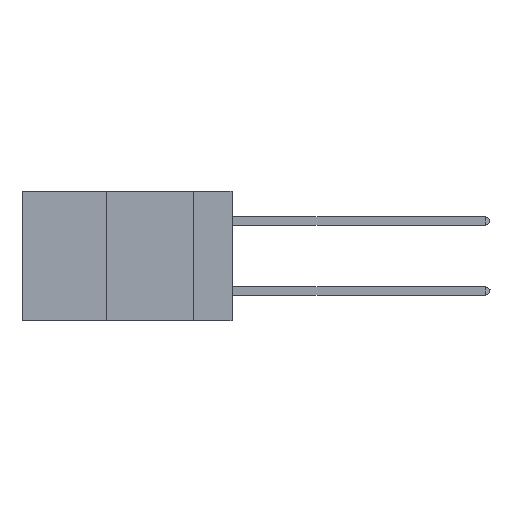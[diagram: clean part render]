
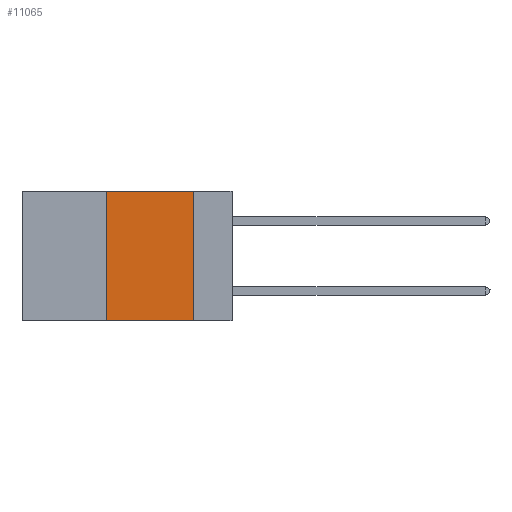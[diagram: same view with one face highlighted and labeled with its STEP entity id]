
A CAD part, left-side view. The second image highlights one B-rep face of the part: STEP entity #11065.
In plain terms, the highlighted planar face has unit normal (-1, 0, 0).
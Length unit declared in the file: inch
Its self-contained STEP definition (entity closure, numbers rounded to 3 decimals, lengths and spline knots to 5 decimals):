
#301 = FACE_OUTER_BOUND ( 'NONE', #7255, .T. ) ;
#517 = CARTESIAN_POINT ( 'NONE',  ( 0., 0.36, 0. ) ) ;
#2562 = DIRECTION ( 'NONE',  ( 0., 0., -1. ) ) ;
#3639 = CARTESIAN_POINT ( 'NONE',  ( 0., 0.36, -0.37 ) ) ;
#3671 = CARTESIAN_POINT ( 'NONE',  ( 0., 0.6, 0. ) ) ;
#3679 = VECTOR ( 'NONE', #15199, 39.37008 ) ;
#4040 = EDGE_CURVE ( 'NONE', #8994, #13096, #10543, .T. ) ;
#5008 = DIRECTION ( 'NONE',  ( 0., -1., 0. ) ) ;
#5077 = CARTESIAN_POINT ( 'NONE',  ( 0., 0.6, 0. ) ) ;
#5802 = DIRECTION ( 'NONE',  ( 0., 0., 1. ) ) ;
#5812 = VERTEX_POINT ( 'NONE', #517 ) ;
#6874 = VECTOR ( 'NONE', #10555, 39.37008 ) ;
#7255 = EDGE_LOOP ( 'NONE', ( #11580, #15272, #14123, #12984 ) ) ;
#7792 = DIRECTION ( 'NONE',  ( 1., 0., 0. ) ) ;
#8140 = LINE ( 'NONE', #3671, #11797 ) ;
#8572 = LINE ( 'NONE', #12608, #3679 ) ;
#8668 = EDGE_CURVE ( 'NONE', #5812, #8994, #8140, .T. ) ;
#8994 = VERTEX_POINT ( 'NONE', #13191 ) ;
#9683 = LINE ( 'NONE', #9754, #10897 ) ;
#9754 = CARTESIAN_POINT ( 'NONE',  ( 0., 0.36, 0. ) ) ;
#10404 = VERTEX_POINT ( 'NONE', #3639 ) ;
#10411 = PLANE ( 'NONE',  #10594 ) ;
#10543 = LINE ( 'NONE', #10613, #6874 ) ;
#10555 = DIRECTION ( 'NONE',  ( 0., 0., -1. ) ) ;
#10594 = AXIS2_PLACEMENT_3D ( 'NONE', #5077, #7792, #2562 ) ;
#10613 = CARTESIAN_POINT ( 'NONE',  ( 0., 0.11, 0. ) ) ;
#10897 = VECTOR ( 'NONE', #5802, 39.37008 ) ;
#11065 = ADVANCED_FACE ( 'NONE', ( #301 ), #10411, .F. ) ;
#11479 = CARTESIAN_POINT ( 'NONE',  ( 0., 0.11, -0.37 ) ) ;
#11580 = ORIENTED_EDGE ( 'NONE', *, *, #4040, .F. ) ;
#11797 = VECTOR ( 'NONE', #5008, 39.37008 ) ;
#11815 = EDGE_CURVE ( 'NONE', #10404, #5812, #9683, .T. ) ;
#12608 = CARTESIAN_POINT ( 'NONE',  ( 0., 0.6, -0.37 ) ) ;
#12984 = ORIENTED_EDGE ( 'NONE', *, *, #14963, .T. ) ;
#13096 = VERTEX_POINT ( 'NONE', #11479 ) ;
#13191 = CARTESIAN_POINT ( 'NONE',  ( 0., 0.11, 0. ) ) ;
#14123 = ORIENTED_EDGE ( 'NONE', *, *, #11815, .F. ) ;
#14963 = EDGE_CURVE ( 'NONE', #10404, #13096, #8572, .T. ) ;
#15199 = DIRECTION ( 'NONE',  ( 0., -1., 0. ) ) ;
#15272 = ORIENTED_EDGE ( 'NONE', *, *, #8668, .F. ) ;
